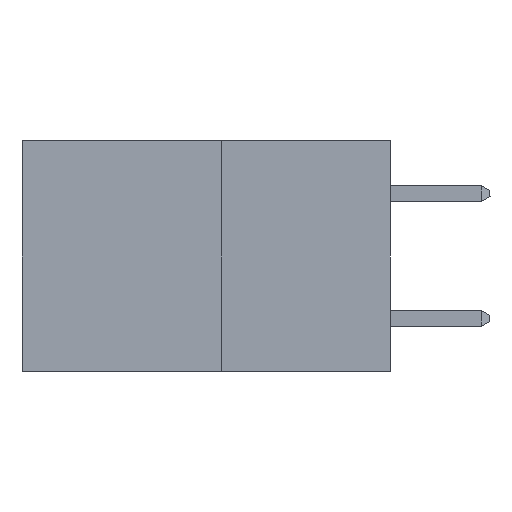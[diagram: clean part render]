
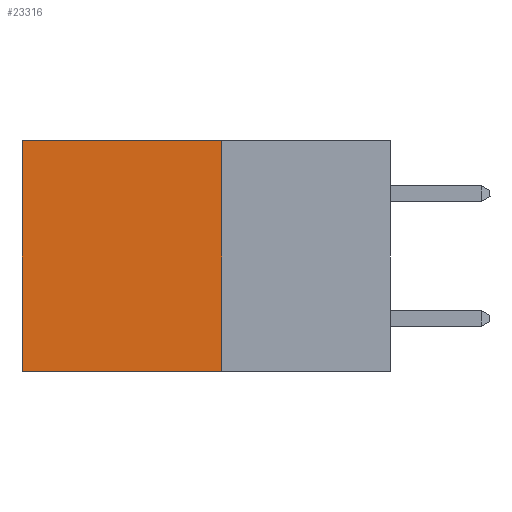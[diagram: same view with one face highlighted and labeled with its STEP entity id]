
A CAD part, left-side view. The second image highlights one B-rep face of the part: STEP entity #23316.
In plain terms, the highlighted planar face has unit normal (-1, 0, 0).
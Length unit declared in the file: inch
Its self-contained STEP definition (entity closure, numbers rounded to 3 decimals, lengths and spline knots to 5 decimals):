
#1836 = ORIENTED_EDGE ( 'NONE', *, *, #17644, .F. ) ;
#3251 = CARTESIAN_POINT ( 'NONE',  ( 0.277, 0.27, 0. ) ) ;
#3270 = VECTOR ( 'NONE', #17314, 39.37008 ) ;
#5152 = ORIENTED_EDGE ( 'NONE', *, *, #19056, .T. ) ;
#5355 = PLANE ( 'NONE',  #31597 ) ;
#5744 = DIRECTION ( 'NONE',  ( 0., 1., 0. ) ) ;
#8420 = LINE ( 'NONE', #9321, #21690 ) ;
#9321 = CARTESIAN_POINT ( 'NONE',  ( 0.277, 0.27, -0.37 ) ) ;
#10159 = CARTESIAN_POINT ( 'NONE',  ( 0.277, 0.27, -0.37 ) ) ;
#10275 = DIRECTION ( 'NONE',  ( 0., 0., -1. ) ) ;
#10588 = LINE ( 'NONE', #29866, #3270 ) ;
#11056 = CARTESIAN_POINT ( 'NONE',  ( 0.277, 0.59, -0.37 ) ) ;
#11532 = CARTESIAN_POINT ( 'NONE',  ( 0.277, 0.59, 0. ) ) ;
#11762 = VERTEX_POINT ( 'NONE', #11532 ) ;
#11789 = DIRECTION ( 'NONE',  ( 0., 1., 0. ) ) ;
#12409 = EDGE_CURVE ( 'NONE', #11762, #14268, #12949, .T. ) ;
#12949 = LINE ( 'NONE', #29197, #24732 ) ;
#14111 = VECTOR ( 'NONE', #5744, 39.37008 ) ;
#14268 = VERTEX_POINT ( 'NONE', #11056 ) ;
#17314 = DIRECTION ( 'NONE',  ( 0., 0., -1. ) ) ;
#17644 = EDGE_CURVE ( 'NONE', #19167, #14268, #8420, .T. ) ;
#18582 = FACE_OUTER_BOUND ( 'NONE', #30354, .T. ) ;
#19056 = EDGE_CURVE ( 'NONE', #19678, #11762, #27451, .T. ) ;
#19167 = VERTEX_POINT ( 'NONE', #20816 ) ;
#19678 = VERTEX_POINT ( 'NONE', #25305 ) ;
#20816 = CARTESIAN_POINT ( 'NONE',  ( 0.277, 0.27, -0.37 ) ) ;
#21690 = VECTOR ( 'NONE', #11789, 39.37008 ) ;
#23316 = ADVANCED_FACE ( 'NONE', ( #18582 ), #5355, .F. ) ;
#24278 = DIRECTION ( 'NONE',  ( 0., 0., -1. ) ) ;
#24732 = VECTOR ( 'NONE', #24278, 39.37008 ) ;
#25305 = CARTESIAN_POINT ( 'NONE',  ( 0.277, 0.27, 0. ) ) ;
#27451 = LINE ( 'NONE', #3251, #14111 ) ;
#27852 = ORIENTED_EDGE ( 'NONE', *, *, #12409, .T. ) ;
#29197 = CARTESIAN_POINT ( 'NONE',  ( 0.277, 0.59, -0.37 ) ) ;
#29866 = CARTESIAN_POINT ( 'NONE',  ( 0.277, 0.27, -0.37 ) ) ;
#30178 = DIRECTION ( 'NONE',  ( 1., 0., 0. ) ) ;
#30354 = EDGE_LOOP ( 'NONE', ( #27852, #1836, #30836, #5152 ) ) ;
#30836 = ORIENTED_EDGE ( 'NONE', *, *, #31974, .F. ) ;
#31597 = AXIS2_PLACEMENT_3D ( 'NONE', #10159, #30178, #10275 ) ;
#31974 = EDGE_CURVE ( 'NONE', #19678, #19167, #10588, .T. ) ;
